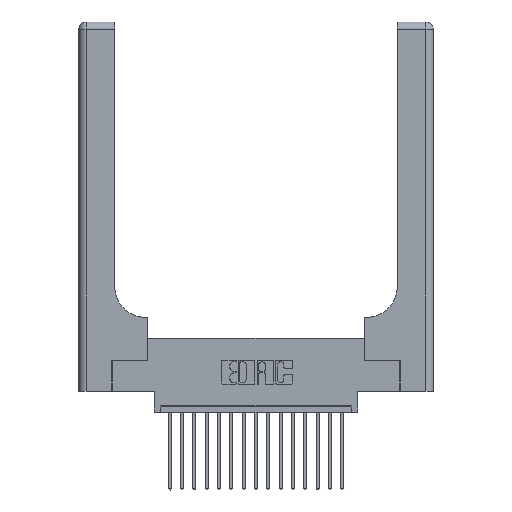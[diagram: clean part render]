
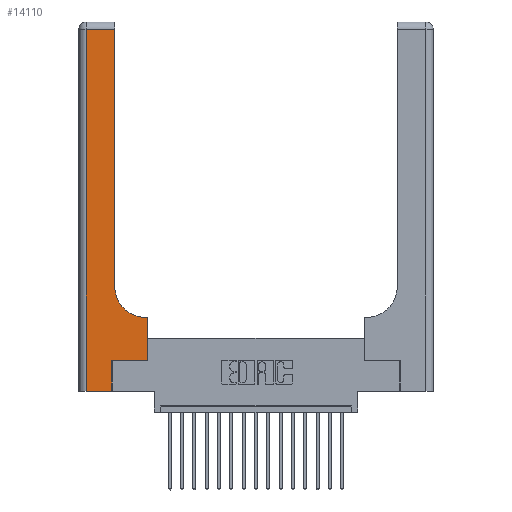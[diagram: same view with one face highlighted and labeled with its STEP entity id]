
A CAD part, top view. The second image highlights one B-rep face of the part: STEP entity #14110.
In plain terms, the highlighted planar face has unit normal (0, 0, 1).
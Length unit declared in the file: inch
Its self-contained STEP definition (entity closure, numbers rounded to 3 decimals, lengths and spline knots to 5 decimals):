
#633 = VECTOR ( 'NONE', #7105, 39.37008 ) ;
#709 = VERTEX_POINT ( 'NONE', #6042 ) ;
#781 = LINE ( 'NONE', #8020, #2267 ) ;
#813 = PLANE ( 'NONE',  #11560 ) ;
#893 = ORIENTED_EDGE ( 'NONE', *, *, #7446, .T. ) ;
#1142 = CARTESIAN_POINT ( 'NONE',  ( 0.5585, 0.25, 0.37 ) ) ;
#1167 = CARTESIAN_POINT ( 'NONE',  ( 0., 0., 0.37 ) ) ;
#1578 = ORIENTED_EDGE ( 'NONE', *, *, #12088, .T. ) ;
#2267 = VECTOR ( 'NONE', #6536, 39.37008 ) ;
#2287 = LINE ( 'NONE', #2752, #10835 ) ;
#2577 = LINE ( 'NONE', #1142, #13068 ) ;
#2675 = VECTOR ( 'NONE', #18771, 39.37008 ) ;
#2752 = CARTESIAN_POINT ( 'NONE',  ( 0., 2.94, 0.37 ) ) ;
#2772 = DIRECTION ( 'NONE',  ( 1., 0., 0. ) ) ;
#2811 = CARTESIAN_POINT ( 'NONE',  ( 0.2915, 2.94, 0.37 ) ) ;
#2813 = ORIENTED_EDGE ( 'NONE', *, *, #15575, .T. ) ;
#2832 = DIRECTION ( 'NONE',  ( -1., 0., 0. ) ) ;
#2962 = VERTEX_POINT ( 'NONE', #20189 ) ;
#3082 = VERTEX_POINT ( 'NONE', #16019 ) ;
#3778 = LINE ( 'NONE', #8685, #13486 ) ;
#4166 = DIRECTION ( 'NONE',  ( 0., 0., -1. ) ) ;
#5431 = CARTESIAN_POINT ( 'NONE',  ( 0.5585, 0.25, 0.37 ) ) ;
#5454 = CARTESIAN_POINT ( 'NONE',  ( 0.2915, 3., 0.37 ) ) ;
#5802 = LINE ( 'NONE', #11719, #12876 ) ;
#6042 = CARTESIAN_POINT ( 'NONE',  ( 0.269, 0., 0.37 ) ) ;
#6458 = EDGE_CURVE ( 'NONE', #18833, #19588, #18437, .T. ) ;
#6536 = DIRECTION ( 'NONE',  ( 0., 1., 0. ) ) ;
#6875 = LINE ( 'NONE', #1167, #18795 ) ;
#6898 = VERTEX_POINT ( 'NONE', #2811 ) ;
#6945 = VERTEX_POINT ( 'NONE', #9731 ) ;
#7105 = DIRECTION ( 'NONE',  ( 0., 1., 0. ) ) ;
#7446 = EDGE_CURVE ( 'NONE', #6898, #6945, #2287, .T. ) ;
#7522 = DIRECTION ( 'NONE',  ( 1., 0., 0. ) ) ;
#7593 = AXIS2_PLACEMENT_3D ( 'NONE', #15513, #17629, #7522 ) ;
#7616 = EDGE_CURVE ( 'NONE', #709, #3082, #781, .T. ) ;
#8020 = CARTESIAN_POINT ( 'NONE',  ( 0.269, 0., 0.37 ) ) ;
#8685 = CARTESIAN_POINT ( 'NONE',  ( 0.2915, 0.6, 0.37 ) ) ;
#8894 = EDGE_CURVE ( 'NONE', #13915, #18833, #3778, .T. ) ;
#9504 = FACE_OUTER_BOUND ( 'NONE', #17430, .T. ) ;
#9731 = CARTESIAN_POINT ( 'NONE',  ( 0.06, 2.94, 0.37 ) ) ;
#10130 = EDGE_CURVE ( 'NONE', #2962, #709, #6875, .T. ) ;
#10426 = VERTEX_POINT ( 'NONE', #5431 ) ;
#10636 = EDGE_CURVE ( 'NONE', #6945, #2962, #15096, .T. ) ;
#10738 = ORIENTED_EDGE ( 'NONE', *, *, #8894, .T. ) ;
#10835 = VECTOR ( 'NONE', #2832, 39.37008 ) ;
#11560 = AXIS2_PLACEMENT_3D ( 'NONE', #13440, #4166, #16572 ) ;
#11628 = ORIENTED_EDGE ( 'NONE', *, *, #14774, .T. ) ;
#11719 = CARTESIAN_POINT ( 'NONE',  ( 0.269, 0.25, 0.37 ) ) ;
#12088 = EDGE_CURVE ( 'NONE', #3082, #10426, #5802, .T. ) ;
#12876 = VECTOR ( 'NONE', #14715, 39.37008 ) ;
#13042 = CARTESIAN_POINT ( 'NONE',  ( 0.2915, 0.85, 0.37 ) ) ;
#13068 = VECTOR ( 'NONE', #16780, 39.37008 ) ;
#13440 = CARTESIAN_POINT ( 'NONE',  ( 0., 3., 0.37 ) ) ;
#13486 = VECTOR ( 'NONE', #16498, 39.37008 ) ;
#13498 = ORIENTED_EDGE ( 'NONE', *, *, #10636, .T. ) ;
#13915 = VERTEX_POINT ( 'NONE', #15699 ) ;
#14110 = ADVANCED_FACE ( 'NONE', ( #9504 ), #813, .F. ) ;
#14715 = DIRECTION ( 'NONE',  ( 1., 0., 0. ) ) ;
#14774 = EDGE_CURVE ( 'NONE', #19588, #6898, #17969, .T. ) ;
#15096 = LINE ( 'NONE', #18983, #2675 ) ;
#15240 = ORIENTED_EDGE ( 'NONE', *, *, #6458, .T. ) ;
#15513 = CARTESIAN_POINT ( 'NONE',  ( 0.5415, 0.85, 0.37 ) ) ;
#15575 = EDGE_CURVE ( 'NONE', #10426, #13915, #2577, .T. ) ;
#15699 = CARTESIAN_POINT ( 'NONE',  ( 0.5585, 0.6, 0.37 ) ) ;
#16019 = CARTESIAN_POINT ( 'NONE',  ( 0.269, 0.25, 0.37 ) ) ;
#16498 = DIRECTION ( 'NONE',  ( -1., 0., 0. ) ) ;
#16572 = DIRECTION ( 'NONE',  ( -1., 0., 0. ) ) ;
#16780 = DIRECTION ( 'NONE',  ( 0., 1., 0. ) ) ;
#17068 = ORIENTED_EDGE ( 'NONE', *, *, #10130, .T. ) ;
#17426 = CARTESIAN_POINT ( 'NONE',  ( 0.5415, 0.6, 0.37 ) ) ;
#17430 = EDGE_LOOP ( 'NONE', ( #11628, #893, #13498, #17068, #20219, #1578, #2813, #10738, #15240 ) ) ;
#17629 = DIRECTION ( 'NONE',  ( 0., 0., -1. ) ) ;
#17969 = LINE ( 'NONE', #5454, #633 ) ;
#18437 = CIRCLE ( 'NONE', #7593, 0.25 ) ;
#18771 = DIRECTION ( 'NONE',  ( 0., -1., 0. ) ) ;
#18795 = VECTOR ( 'NONE', #2772, 39.37008 ) ;
#18833 = VERTEX_POINT ( 'NONE', #17426 ) ;
#18983 = CARTESIAN_POINT ( 'NONE',  ( 0.06, 3., 0.37 ) ) ;
#19588 = VERTEX_POINT ( 'NONE', #13042 ) ;
#20189 = CARTESIAN_POINT ( 'NONE',  ( 0.06, 0., 0.37 ) ) ;
#20219 = ORIENTED_EDGE ( 'NONE', *, *, #7616, .T. ) ;
